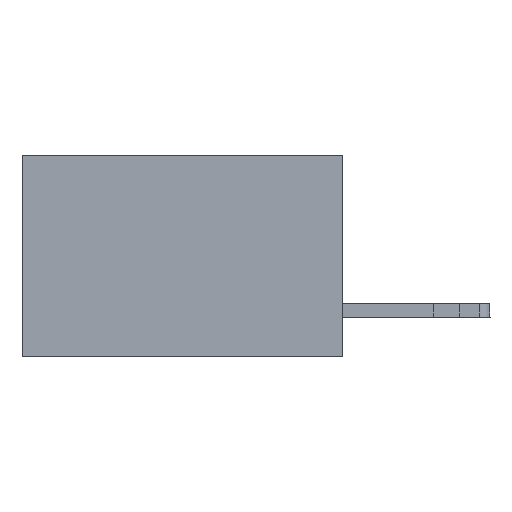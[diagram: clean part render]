
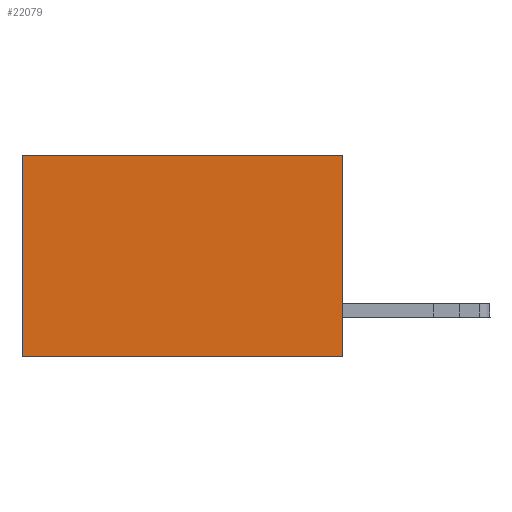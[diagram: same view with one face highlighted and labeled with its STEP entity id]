
A CAD part, left-side view. The second image highlights one B-rep face of the part: STEP entity #22079.
In plain terms, the highlighted planar face has unit normal (-1, 0, 0).
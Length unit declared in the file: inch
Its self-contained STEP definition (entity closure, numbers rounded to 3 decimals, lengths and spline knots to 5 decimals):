
#728 = EDGE_LOOP ( 'NONE', ( #14902, #21407, #22271, #18138 ) ) ;
#1293 = AXIS2_PLACEMENT_3D ( 'NONE', #11629, #28075, #13993 ) ;
#3845 = VECTOR ( 'NONE', #9983, 39.37008 ) ;
#4932 = VERTEX_POINT ( 'NONE', #21032 ) ;
#6821 = VECTOR ( 'NONE', #26597, 39.37008 ) ;
#6854 = VECTOR ( 'NONE', #15492, 39.37008 ) ;
#9316 = VECTOR ( 'NONE', #14898, 39.37008 ) ;
#9445 = LINE ( 'NONE', #24098, #3845 ) ;
#9983 = DIRECTION ( 'NONE',  ( 0., 1., 0. ) ) ;
#10059 = LINE ( 'NONE', #26642, #9316 ) ;
#10426 = CARTESIAN_POINT ( 'NONE',  ( 0.277, 0., -0.37 ) ) ;
#11629 = CARTESIAN_POINT ( 'NONE',  ( 0.277, 0., -0.37 ) ) ;
#12041 = VERTEX_POINT ( 'NONE', #16525 ) ;
#13110 = LINE ( 'NONE', #19529, #6821 ) ;
#13993 = DIRECTION ( 'NONE',  ( 0., 0., -1. ) ) ;
#14898 = DIRECTION ( 'NONE',  ( 0., 0., -1. ) ) ;
#14902 = ORIENTED_EDGE ( 'NONE', *, *, #18570, .T. ) ;
#15492 = DIRECTION ( 'NONE',  ( 0., 1., 0. ) ) ;
#16525 = CARTESIAN_POINT ( 'NONE',  ( 0.277, 0.59, -0.37 ) ) ;
#17214 = LINE ( 'NONE', #29527, #6854 ) ;
#18138 = ORIENTED_EDGE ( 'NONE', *, *, #27137, .T. ) ;
#18570 = EDGE_CURVE ( 'NONE', #4932, #12041, #13110, .T. ) ;
#19409 = FACE_OUTER_BOUND ( 'NONE', #728, .T. ) ;
#19529 = CARTESIAN_POINT ( 'NONE',  ( 0.277, 0.59, -0.37 ) ) ;
#20439 = EDGE_CURVE ( 'NONE', #28566, #29073, #10059, .T. ) ;
#21032 = CARTESIAN_POINT ( 'NONE',  ( 0.277, 0.59, 0. ) ) ;
#21407 = ORIENTED_EDGE ( 'NONE', *, *, #28259, .F. ) ;
#22079 = ADVANCED_FACE ( 'NONE', ( #19409 ), #27967, .F. ) ;
#22271 = ORIENTED_EDGE ( 'NONE', *, *, #20439, .F. ) ;
#24098 = CARTESIAN_POINT ( 'NONE',  ( 0.277, 0., -0.37 ) ) ;
#26597 = DIRECTION ( 'NONE',  ( 0., 0., -1. ) ) ;
#26642 = CARTESIAN_POINT ( 'NONE',  ( 0.277, 0., -0.37 ) ) ;
#27137 = EDGE_CURVE ( 'NONE', #28566, #4932, #17214, .T. ) ;
#27967 = PLANE ( 'NONE',  #1293 ) ;
#28075 = DIRECTION ( 'NONE',  ( 1., 0., 0. ) ) ;
#28259 = EDGE_CURVE ( 'NONE', #29073, #12041, #9445, .T. ) ;
#28566 = VERTEX_POINT ( 'NONE', #29726 ) ;
#29073 = VERTEX_POINT ( 'NONE', #10426 ) ;
#29527 = CARTESIAN_POINT ( 'NONE',  ( 0.277, 0., 0. ) ) ;
#29726 = CARTESIAN_POINT ( 'NONE',  ( 0.277, 0., 0. ) ) ;
